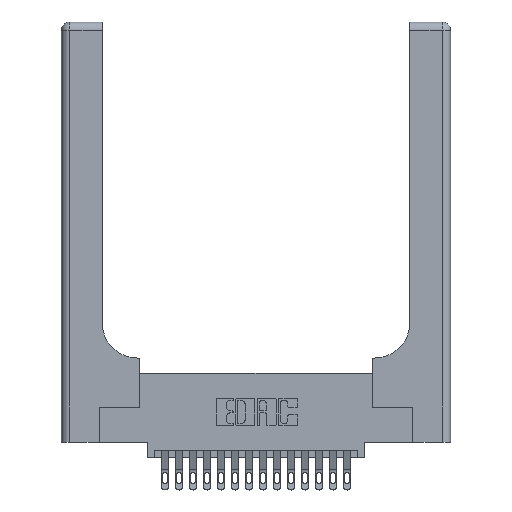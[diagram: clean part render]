
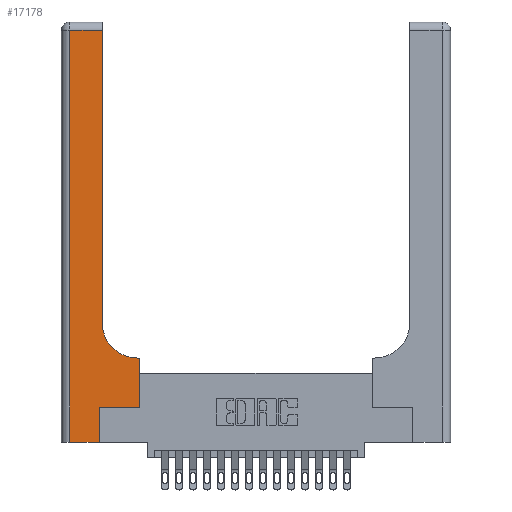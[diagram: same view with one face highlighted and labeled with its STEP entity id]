
A CAD part, top view. The second image highlights one B-rep face of the part: STEP entity #17178.
In plain terms, the highlighted planar face has unit normal (0, 0, 1).
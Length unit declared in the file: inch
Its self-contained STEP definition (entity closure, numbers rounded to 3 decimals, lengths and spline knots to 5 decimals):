
#531 = CARTESIAN_POINT ( 'NONE',  ( 0., 0., 0.37 ) ) ;
#651 = VERTEX_POINT ( 'NONE', #17302 ) ;
#725 = LINE ( 'NONE', #11288, #5644 ) ;
#948 = VECTOR ( 'NONE', #8436, 39.37008 ) ;
#965 = EDGE_CURVE ( 'NONE', #16265, #19911, #17403, .T. ) ;
#1233 = ORIENTED_EDGE ( 'NONE', *, *, #10824, .T. ) ;
#1315 = ORIENTED_EDGE ( 'NONE', *, *, #5234, .T. ) ;
#1464 = ORIENTED_EDGE ( 'NONE', *, *, #965, .T. ) ;
#1515 = AXIS2_PLACEMENT_3D ( 'NONE', #8633, #19393, #10211 ) ;
#1573 = DIRECTION ( 'NONE',  ( 0., 1., 0. ) ) ;
#1588 = EDGE_LOOP ( 'NONE', ( #1233, #2591, #7506, #3646, #19429, #1315, #5643, #1464, #6299 ) ) ;
#2591 = ORIENTED_EDGE ( 'NONE', *, *, #4361, .T. ) ;
#2806 = DIRECTION ( 'NONE',  ( -1., 0., 0. ) ) ;
#2943 = CARTESIAN_POINT ( 'NONE',  ( 0.2915, 0.6, 0.37 ) ) ;
#3646 = ORIENTED_EDGE ( 'NONE', *, *, #4389, .T. ) ;
#3878 = DIRECTION ( 'NONE',  ( 1., 0., 0. ) ) ;
#4031 = CARTESIAN_POINT ( 'NONE',  ( 0.2915, 3., 0.37 ) ) ;
#4141 = CARTESIAN_POINT ( 'NONE',  ( 0.269, 0., 0.37 ) ) ;
#4361 = EDGE_CURVE ( 'NONE', #8431, #18212, #12352, .T. ) ;
#4389 = EDGE_CURVE ( 'NONE', #651, #16982, #15455, .T. ) ;
#4704 = PLANE ( 'NONE',  #15317 ) ;
#4855 = VECTOR ( 'NONE', #16406, 39.37008 ) ;
#5234 = EDGE_CURVE ( 'NONE', #18785, #16694, #18087, .T. ) ;
#5474 = CARTESIAN_POINT ( 'NONE',  ( 0.06, 3., 0.37 ) ) ;
#5643 = ORIENTED_EDGE ( 'NONE', *, *, #16579, .T. ) ;
#5644 = VECTOR ( 'NONE', #1573, 39.37008 ) ;
#6194 = CARTESIAN_POINT ( 'NONE',  ( 0.269, 0.25, 0.37 ) ) ;
#6299 = ORIENTED_EDGE ( 'NONE', *, *, #13255, .T. ) ;
#7150 = VECTOR ( 'NONE', #3878, 39.37008 ) ;
#7506 = ORIENTED_EDGE ( 'NONE', *, *, #17351, .T. ) ;
#7669 = VECTOR ( 'NONE', #8690, 39.37008 ) ;
#7944 = CARTESIAN_POINT ( 'NONE',  ( 0., 3., 0.37 ) ) ;
#8225 = CARTESIAN_POINT ( 'NONE',  ( 0.269, 0., 0.37 ) ) ;
#8265 = VERTEX_POINT ( 'NONE', #17948 ) ;
#8431 = VERTEX_POINT ( 'NONE', #16730 ) ;
#8436 = DIRECTION ( 'NONE',  ( 0., 1., 0. ) ) ;
#8633 = CARTESIAN_POINT ( 'NONE',  ( 0.5415, 0.85, 0.37 ) ) ;
#8690 = DIRECTION ( 'NONE',  ( -1., 0., 0. ) ) ;
#9160 = LINE ( 'NONE', #8225, #948 ) ;
#9234 = VECTOR ( 'NONE', #2806, 39.37008 ) ;
#9435 = VECTOR ( 'NONE', #15560, 39.37008 ) ;
#9570 = DIRECTION ( 'NONE',  ( -1., 0., 0. ) ) ;
#10211 = DIRECTION ( 'NONE',  ( 1., 0., 0. ) ) ;
#10824 = EDGE_CURVE ( 'NONE', #8265, #8431, #14858, .T. ) ;
#11208 = CARTESIAN_POINT ( 'NONE',  ( 0.5415, 0.6, 0.37 ) ) ;
#11288 = CARTESIAN_POINT ( 'NONE',  ( 0.5585, 0.25, 0.37 ) ) ;
#11315 = CARTESIAN_POINT ( 'NONE',  ( 0.269, 0.25, 0.37 ) ) ;
#12313 = LINE ( 'NONE', #5474, #4855 ) ;
#12352 = LINE ( 'NONE', #14851, #7669 ) ;
#12640 = CIRCLE ( 'NONE', #1515, 0.25 ) ;
#12691 = CARTESIAN_POINT ( 'NONE',  ( 0.06, 2.94, 0.37 ) ) ;
#13031 = CARTESIAN_POINT ( 'NONE',  ( 0.5585, 0.25, 0.37 ) ) ;
#13255 = EDGE_CURVE ( 'NONE', #19911, #8265, #12640, .T. ) ;
#13523 = DIRECTION ( 'NONE',  ( 0., 1., 0. ) ) ;
#14851 = CARTESIAN_POINT ( 'NONE',  ( 0., 2.94, 0.37 ) ) ;
#14858 = LINE ( 'NONE', #4031, #18902 ) ;
#15317 = AXIS2_PLACEMENT_3D ( 'NONE', #7944, #18744, #9570 ) ;
#15455 = LINE ( 'NONE', #531, #7150 ) ;
#15560 = DIRECTION ( 'NONE',  ( 1., 0., 0. ) ) ;
#15656 = FACE_OUTER_BOUND ( 'NONE', #1588, .T. ) ;
#16265 = VERTEX_POINT ( 'NONE', #19511 ) ;
#16406 = DIRECTION ( 'NONE',  ( 0., -1., 0. ) ) ;
#16579 = EDGE_CURVE ( 'NONE', #16694, #16265, #725, .T. ) ;
#16694 = VERTEX_POINT ( 'NONE', #13031 ) ;
#16730 = CARTESIAN_POINT ( 'NONE',  ( 0.2915, 2.94, 0.37 ) ) ;
#16982 = VERTEX_POINT ( 'NONE', #4141 ) ;
#17178 = ADVANCED_FACE ( 'NONE', ( #15656 ), #4704, .F. ) ;
#17302 = CARTESIAN_POINT ( 'NONE',  ( 0.06, 0., 0.37 ) ) ;
#17320 = EDGE_CURVE ( 'NONE', #16982, #18785, #9160, .T. ) ;
#17351 = EDGE_CURVE ( 'NONE', #18212, #651, #12313, .T. ) ;
#17403 = LINE ( 'NONE', #2943, #9234 ) ;
#17948 = CARTESIAN_POINT ( 'NONE',  ( 0.2915, 0.85, 0.37 ) ) ;
#18087 = LINE ( 'NONE', #6194, #9435 ) ;
#18212 = VERTEX_POINT ( 'NONE', #12691 ) ;
#18744 = DIRECTION ( 'NONE',  ( 0., 0., -1. ) ) ;
#18785 = VERTEX_POINT ( 'NONE', #11315 ) ;
#18902 = VECTOR ( 'NONE', #13523, 39.37008 ) ;
#19393 = DIRECTION ( 'NONE',  ( 0., 0., -1. ) ) ;
#19429 = ORIENTED_EDGE ( 'NONE', *, *, #17320, .T. ) ;
#19511 = CARTESIAN_POINT ( 'NONE',  ( 0.5585, 0.6, 0.37 ) ) ;
#19911 = VERTEX_POINT ( 'NONE', #11208 ) ;
